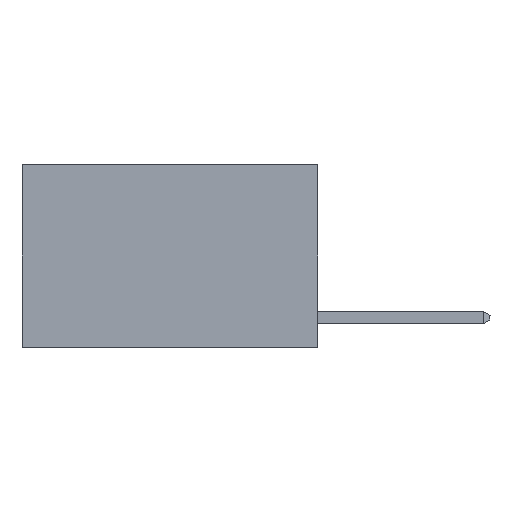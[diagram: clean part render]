
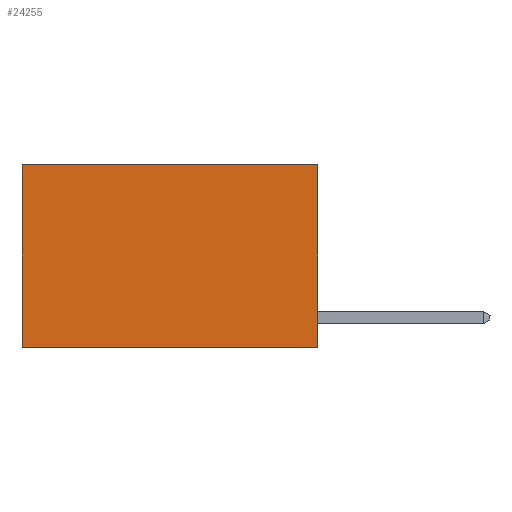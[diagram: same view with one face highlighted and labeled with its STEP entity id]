
A CAD part, left-side view. The second image highlights one B-rep face of the part: STEP entity #24255.
In plain terms, the highlighted planar face has unit normal (-1, 0, 0).
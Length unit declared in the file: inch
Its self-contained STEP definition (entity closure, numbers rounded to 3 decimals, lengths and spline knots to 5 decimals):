
#152 = ORIENTED_EDGE ( 'NONE', *, *, #10827, .T. ) ;
#377 = ORIENTED_EDGE ( 'NONE', *, *, #1579, .T. ) ;
#422 = CARTESIAN_POINT ( 'NONE',  ( 0.2625, 0., -0.37 ) ) ;
#1066 = CARTESIAN_POINT ( 'NONE',  ( 0.2625, 0.6, -0.37 ) ) ;
#1461 = VERTEX_POINT ( 'NONE', #9700 ) ;
#1579 = EDGE_CURVE ( 'NONE', #15230, #14884, #16041, .T. ) ;
#2870 = EDGE_LOOP ( 'NONE', ( #377, #4118, #14858, #152 ) ) ;
#3460 = EDGE_CURVE ( 'NONE', #1461, #14884, #22059, .T. ) ;
#3918 = CARTESIAN_POINT ( 'NONE',  ( 0.2625, 0., 0. ) ) ;
#4118 = ORIENTED_EDGE ( 'NONE', *, *, #3460, .F. ) ;
#6172 = DIRECTION ( 'NONE',  ( 0., 0., -1. ) ) ;
#8254 = LINE ( 'NONE', #10786, #14820 ) ;
#8731 = CARTESIAN_POINT ( 'NONE',  ( 0.2625, 0., 0. ) ) ;
#9378 = VECTOR ( 'NONE', #6172, 39.37008 ) ;
#9700 = CARTESIAN_POINT ( 'NONE',  ( 0.2625, 0., -0.37 ) ) ;
#10487 = VECTOR ( 'NONE', #15466, 39.37008 ) ;
#10786 = CARTESIAN_POINT ( 'NONE',  ( 0.2625, 0., 0. ) ) ;
#10827 = EDGE_CURVE ( 'NONE', #26394, #15230, #19427, .T. ) ;
#11055 = VECTOR ( 'NONE', #25855, 39.37008 ) ;
#12675 = AXIS2_PLACEMENT_3D ( 'NONE', #3918, #21093, #16872 ) ;
#14554 = CARTESIAN_POINT ( 'NONE',  ( 0.2625, 0.6, 0. ) ) ;
#14634 = PLANE ( 'NONE',  #12675 ) ;
#14820 = VECTOR ( 'NONE', #16691, 39.37008 ) ;
#14858 = ORIENTED_EDGE ( 'NONE', *, *, #16679, .F. ) ;
#14884 = VERTEX_POINT ( 'NONE', #1066 ) ;
#15230 = VERTEX_POINT ( 'NONE', #14554 ) ;
#15466 = DIRECTION ( 'NONE',  ( 0., 1., 0. ) ) ;
#16041 = LINE ( 'NONE', #23330, #9378 ) ;
#16679 = EDGE_CURVE ( 'NONE', #26394, #1461, #8254, .T. ) ;
#16691 = DIRECTION ( 'NONE',  ( 0., 0., -1. ) ) ;
#16872 = DIRECTION ( 'NONE',  ( 0., 0., -1. ) ) ;
#19427 = LINE ( 'NONE', #8731, #11055 ) ;
#21093 = DIRECTION ( 'NONE',  ( 1., 0., 0. ) ) ;
#22059 = LINE ( 'NONE', #422, #10487 ) ;
#23330 = CARTESIAN_POINT ( 'NONE',  ( 0.2625, 0.6, 0. ) ) ;
#24255 = ADVANCED_FACE ( 'NONE', ( #27550 ), #14634, .F. ) ;
#24886 = CARTESIAN_POINT ( 'NONE',  ( 0.2625, 0., 0. ) ) ;
#25855 = DIRECTION ( 'NONE',  ( 0., 1., 0. ) ) ;
#26394 = VERTEX_POINT ( 'NONE', #24886 ) ;
#27550 = FACE_OUTER_BOUND ( 'NONE', #2870, .T. ) ;
